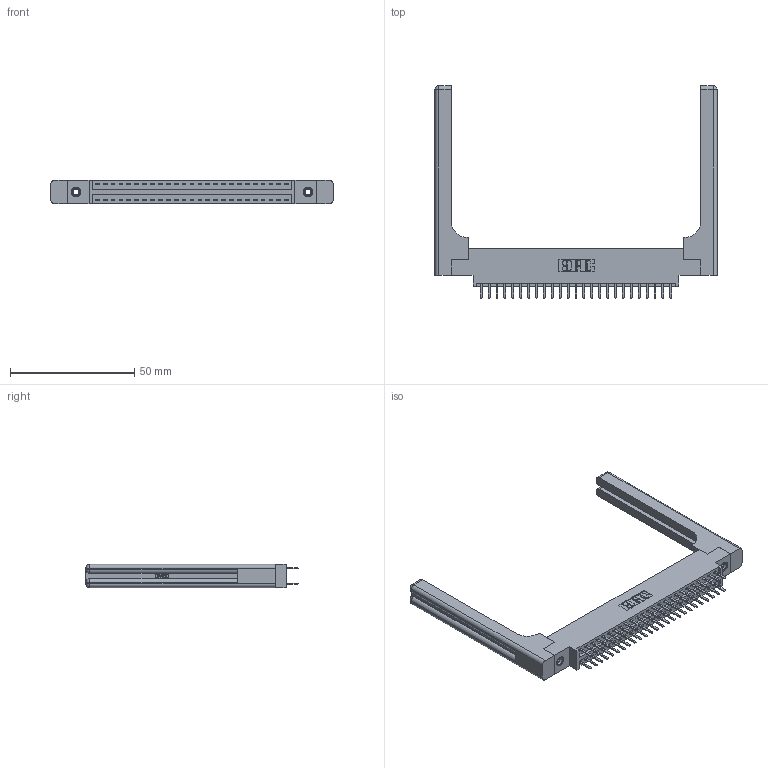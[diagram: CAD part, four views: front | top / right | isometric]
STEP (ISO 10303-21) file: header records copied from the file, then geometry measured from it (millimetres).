
FILE_DESCRIPTION (( 'STEP AP203' ), '1' );
FILE_NAME ('396-050-520-858.STEP', '2019-11-02T07:13:01', ( '' ), ( '' ), 'SwSTEP 2.0', 'SolidWorks 2016', '' );
FILE_SCHEMA (( 'CONFIG_CONTROL_DESIGN' ));
Length unit declared in the file: inch
Products named in the file (5): 396-050-520-858; 346 Part_0.170 Offset - 0.156 Dia-TH; 345-292-001_345-293-120; 345-250-001_345-250-001-102; 346-220-058_345-220-058
Assembly tree (55 placements, depth 2):
  396-050-520-858
    346 Part_0.170 Offset - 0.156 Dia-TH
    345-292-001_345-293-120  x50
    345-250-001_345-250-001-102  x2
    346-220-058_345-220-058  x2
Bounding box: 113.44 x 85.29 x 9.4 mm (x, y, z)
Volume: 18247.1 mm3; surface area: 19614.2 mm2
Topology: 55 solids, 55 shells, 3182 faces, 9157 edges, 5950 vertices
Faces by surface type: plane 2078, cylinder 1044, bspline 36, cone 12, sphere 8, torus 4
Entity records: 24032 total; most frequent: CARTESIAN_POINT 5005, ORIENTED_EDGE 3724, DIRECTION 3382, EDGE_CURVE 1862, VECTOR 1534, LINE 1534, VERTEX_POINT 1230, AXIS2_PLACEMENT_3D 924
